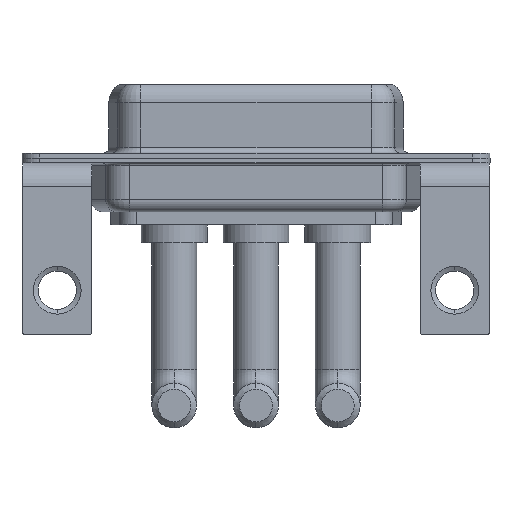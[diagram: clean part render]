
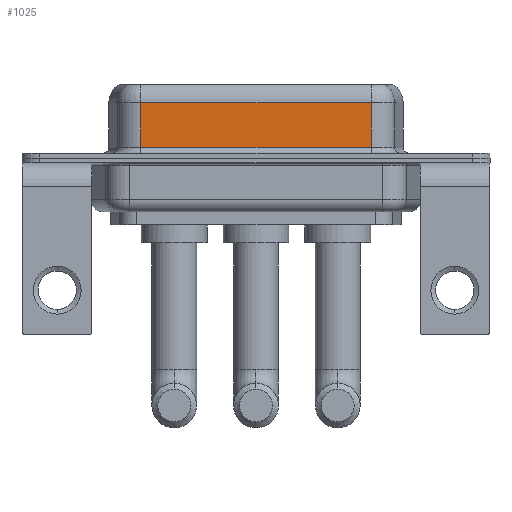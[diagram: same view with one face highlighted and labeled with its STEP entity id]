
A CAD part, front view. The second image highlights one B-rep face of the part: STEP entity #1025.
In plain terms, the highlighted planar face has unit normal (0, -1, 0).
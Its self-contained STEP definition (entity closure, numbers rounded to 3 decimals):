
#238 = LINE ( 'NONE', #4592, #6259 ) ;
#553 = DIRECTION ( 'NONE',  ( -1., 0., 0. ) ) ;
#1025 = ADVANCED_FACE ( 'NONE', ( #3343 ), #3407, .F. ) ;
#1268 = ORIENTED_EDGE ( 'NONE', *, *, #11732, .T. ) ;
#1607 = DIRECTION ( 'NONE',  ( 1., 0., 0. ) ) ;
#1680 = LINE ( 'NONE', #2549, #9252 ) ;
#1809 = ORIENTED_EDGE ( 'NONE', *, *, #3151, .F. ) ;
#2315 = CARTESIAN_POINT ( 'NONE',  ( 7.013, -3.95, 6.4 ) ) ;
#2379 = LINE ( 'NONE', #2315, #5096 ) ;
#2440 = ORIENTED_EDGE ( 'NONE', *, *, #5924, .T. ) ;
#2549 = CARTESIAN_POINT ( 'NONE',  ( 26.287, -3.95, 4.65 ) ) ;
#2840 = VERTEX_POINT ( 'NONE', #12241 ) ;
#3151 = EDGE_CURVE ( 'NONE', #2840, #6739, #11072, .T. ) ;
#3343 = FACE_OUTER_BOUND ( 'NONE', #7168, .T. ) ;
#3407 = PLANE ( 'NONE',  #9831 ) ;
#4592 = CARTESIAN_POINT ( 'NONE',  ( 26.287, -3.95, 0.9 ) ) ;
#5096 = VECTOR ( 'NONE', #10381, 1000. ) ;
#5574 = CARTESIAN_POINT ( 'NONE',  ( 7.013, -3.95, 0.9 ) ) ;
#5924 = EDGE_CURVE ( 'NONE', #7388, #6739, #238, .T. ) ;
#6259 = VECTOR ( 'NONE', #1607, 1000. ) ;
#6739 = VERTEX_POINT ( 'NONE', #7124 ) ;
#6804 = EDGE_CURVE ( 'NONE', #8200, #7388, #2379, .T. ) ;
#7050 = CARTESIAN_POINT ( 'NONE',  ( 7.013, -3.95, 4.65 ) ) ;
#7124 = CARTESIAN_POINT ( 'NONE',  ( 26.287, -3.95, 0.9 ) ) ;
#7168 = EDGE_LOOP ( 'NONE', ( #1809, #1268, #7679, #2440 ) ) ;
#7388 = VERTEX_POINT ( 'NONE', #5574 ) ;
#7679 = ORIENTED_EDGE ( 'NONE', *, *, #6804, .T. ) ;
#7842 = DIRECTION ( 'NONE',  ( 0., 0., -1. ) ) ;
#8200 = VERTEX_POINT ( 'NONE', #7050 ) ;
#8858 = VECTOR ( 'NONE', #7842, 1000. ) ;
#9252 = VECTOR ( 'NONE', #553, 1000. ) ;
#9831 = AXIS2_PLACEMENT_3D ( 'NONE', #10154, #12495, #10277 ) ;
#10154 = CARTESIAN_POINT ( 'NONE',  ( 26.287, -3.95, 6.4 ) ) ;
#10277 = DIRECTION ( 'NONE',  ( 0., 0., 1. ) ) ;
#10381 = DIRECTION ( 'NONE',  ( 0., 0., -1. ) ) ;
#11072 = LINE ( 'NONE', #12972, #8858 ) ;
#11732 = EDGE_CURVE ( 'NONE', #2840, #8200, #1680, .T. ) ;
#12241 = CARTESIAN_POINT ( 'NONE',  ( 26.287, -3.95, 4.65 ) ) ;
#12495 = DIRECTION ( 'NONE',  ( 0., 1., 0. ) ) ;
#12972 = CARTESIAN_POINT ( 'NONE',  ( 26.287, -3.95, 6.4 ) ) ;
